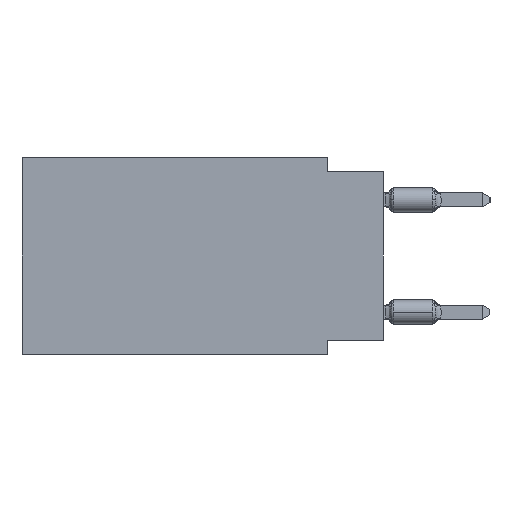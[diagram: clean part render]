
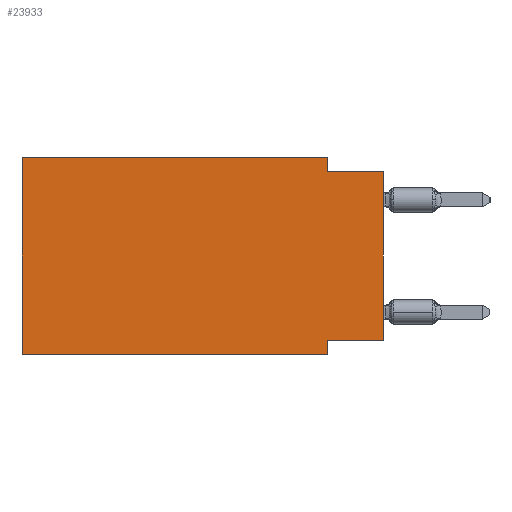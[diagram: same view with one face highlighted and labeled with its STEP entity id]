
A CAD part, left-side view. The second image highlights one B-rep face of the part: STEP entity #23933.
In plain terms, the highlighted planar face has unit normal (-1, 0, 0).
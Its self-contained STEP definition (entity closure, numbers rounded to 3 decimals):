
#1596 = CARTESIAN_POINT ( 'NONE',  ( 0., 2.54, -0.635 ) ) ;
#2687 = ORIENTED_EDGE ( 'NONE', *, *, #13673, .F. ) ;
#3369 = DIRECTION ( 'NONE',  ( 1., 0., 0. ) ) ;
#5526 = DIRECTION ( 'NONE',  ( 0., -1., 0. ) ) ;
#6874 = ORIENTED_EDGE ( 'NONE', *, *, #37141, .F. ) ;
#8586 = CARTESIAN_POINT ( 'NONE',  ( 0., 2.54, -8.89 ) ) ;
#8700 = DIRECTION ( 'NONE',  ( 0., 0., 1. ) ) ;
#8968 = LINE ( 'NONE', #32282, #25625 ) ;
#9288 = VECTOR ( 'NONE', #27827, 1000. ) ;
#9625 = LINE ( 'NONE', #26300, #38316 ) ;
#10052 = DIRECTION ( 'NONE',  ( 0., 1., 0. ) ) ;
#10883 = EDGE_CURVE ( 'NONE', #38493, #48039, #30328, .T. ) ;
#13673 = EDGE_CURVE ( 'NONE', #48039, #35870, #18872, .T. ) ;
#14838 = CARTESIAN_POINT ( 'NONE',  ( 0., 16.383, 0. ) ) ;
#15495 = ORIENTED_EDGE ( 'NONE', *, *, #41773, .T. ) ;
#15821 = VERTEX_POINT ( 'NONE', #42489 ) ;
#15864 = CARTESIAN_POINT ( 'NONE',  ( 0., 0., -0.635 ) ) ;
#16558 = VECTOR ( 'NONE', #10052, 1000. ) ;
#16731 = DIRECTION ( 'NONE',  ( 0., 0., -1. ) ) ;
#17639 = VERTEX_POINT ( 'NONE', #15864 ) ;
#18222 = CARTESIAN_POINT ( 'NONE',  ( 0., 2.54, 0. ) ) ;
#18278 = ORIENTED_EDGE ( 'NONE', *, *, #53597, .F. ) ;
#18872 = LINE ( 'NONE', #31727, #42123 ) ;
#19387 = EDGE_CURVE ( 'NONE', #33195, #35870, #23375, .T. ) ;
#23103 = DIRECTION ( 'NONE',  ( 0., -1., 0. ) ) ;
#23320 = DIRECTION ( 'NONE',  ( 0., 0., -1. ) ) ;
#23375 = LINE ( 'NONE', #27472, #24072 ) ;
#23933 = ADVANCED_FACE ( 'NONE', ( #39997 ), #48198, .F. ) ;
#24016 = CARTESIAN_POINT ( 'NONE',  ( 0., 0., 0. ) ) ;
#24072 = VECTOR ( 'NONE', #23103, 1000. ) ;
#24455 = ORIENTED_EDGE ( 'NONE', *, *, #10883, .F. ) ;
#24524 = CARTESIAN_POINT ( 'NONE',  ( 0., 0., -0.635 ) ) ;
#25625 = VECTOR ( 'NONE', #8700, 1000. ) ;
#26243 = EDGE_CURVE ( 'NONE', #15821, #32643, #9625, .T. ) ;
#26300 = CARTESIAN_POINT ( 'NONE',  ( 0., 16.383, 0. ) ) ;
#27429 = CARTESIAN_POINT ( 'NONE',  ( 0., 16.383, -8.89 ) ) ;
#27472 = CARTESIAN_POINT ( 'NONE',  ( 0., 16.383, -8.89 ) ) ;
#27827 = DIRECTION ( 'NONE',  ( 0., 0., 1. ) ) ;
#28906 = ORIENTED_EDGE ( 'NONE', *, *, #19387, .T. ) ;
#29924 = AXIS2_PLACEMENT_3D ( 'NONE', #14838, #3369, #23320 ) ;
#30117 = ORIENTED_EDGE ( 'NONE', *, *, #33899, .F. ) ;
#30328 = LINE ( 'NONE', #35208, #16558 ) ;
#31727 = CARTESIAN_POINT ( 'NONE',  ( 0., 2.54, -8.89 ) ) ;
#32282 = CARTESIAN_POINT ( 'NONE',  ( 0., 16.383, 0. ) ) ;
#32643 = VERTEX_POINT ( 'NONE', #18222 ) ;
#33195 = VERTEX_POINT ( 'NONE', #27429 ) ;
#33899 = EDGE_CURVE ( 'NONE', #33195, #15821, #8968, .T. ) ;
#35063 = VECTOR ( 'NONE', #16731, 1000. ) ;
#35208 = CARTESIAN_POINT ( 'NONE',  ( 0., 0., -8.255 ) ) ;
#35870 = VERTEX_POINT ( 'NONE', #8586 ) ;
#37141 = EDGE_CURVE ( 'NONE', #41413, #17639, #53769, .T. ) ;
#38316 = VECTOR ( 'NONE', #5526, 1000. ) ;
#38493 = VERTEX_POINT ( 'NONE', #51690 ) ;
#39747 = ORIENTED_EDGE ( 'NONE', *, *, #26243, .F. ) ;
#39997 = FACE_OUTER_BOUND ( 'NONE', #44283, .T. ) ;
#41208 = DIRECTION ( 'NONE',  ( 0., -1., 0. ) ) ;
#41413 = VERTEX_POINT ( 'NONE', #1596 ) ;
#41630 = CARTESIAN_POINT ( 'NONE',  ( 0., 2.54, 0. ) ) ;
#41773 = EDGE_CURVE ( 'NONE', #38493, #17639, #45348, .T. ) ;
#42123 = VECTOR ( 'NONE', #44021, 1000. ) ;
#42489 = CARTESIAN_POINT ( 'NONE',  ( 0., 16.383, 0. ) ) ;
#43598 = CARTESIAN_POINT ( 'NONE',  ( 0., 2.54, -8.255 ) ) ;
#44021 = DIRECTION ( 'NONE',  ( 0., 0., -1. ) ) ;
#44283 = EDGE_LOOP ( 'NONE', ( #15495, #6874, #18278, #39747, #30117, #28906, #2687, #24455 ) ) ;
#45348 = LINE ( 'NONE', #24016, #9288 ) ;
#45456 = LINE ( 'NONE', #41630, #35063 ) ;
#48039 = VERTEX_POINT ( 'NONE', #43598 ) ;
#48198 = PLANE ( 'NONE',  #29924 ) ;
#51690 = CARTESIAN_POINT ( 'NONE',  ( 0., 0., -8.255 ) ) ;
#52811 = VECTOR ( 'NONE', #41208, 1000. ) ;
#53597 = EDGE_CURVE ( 'NONE', #32643, #41413, #45456, .T. ) ;
#53769 = LINE ( 'NONE', #24524, #52811 ) ;
